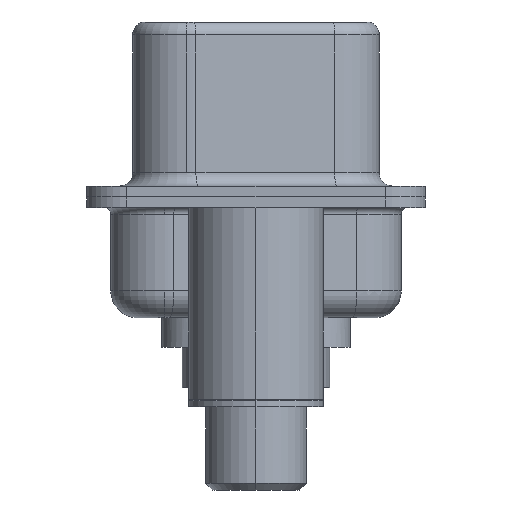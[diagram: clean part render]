
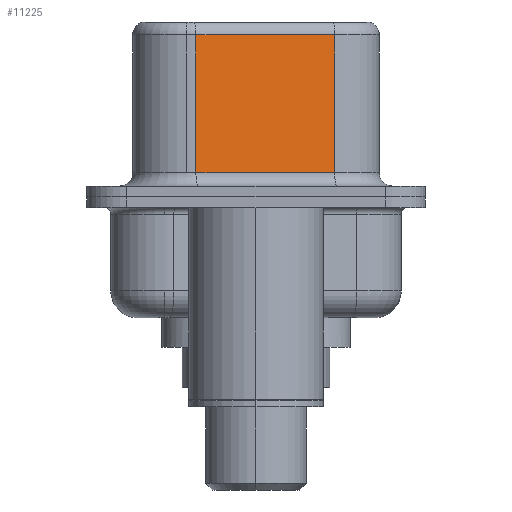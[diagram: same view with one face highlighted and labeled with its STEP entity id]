
A CAD part, left-side view. The second image highlights one B-rep face of the part: STEP entity #11225.
In plain terms, the highlighted planar face has unit normal (-0.985, -0.174, 0).
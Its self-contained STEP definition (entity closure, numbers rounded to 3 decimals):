
#11 = ORIENTED_EDGE ( 'NONE', *, *, #8225, .T. ) ;
#1440 = CARTESIAN_POINT ( 'NONE',  ( 4.565, -2.927, 0.9 ) ) ;
#1523 = VERTEX_POINT ( 'NONE', #1440 ) ;
#1738 = LINE ( 'NONE', #8258, #13459 ) ;
#1987 = LINE ( 'NONE', #2296, #6520 ) ;
#2296 = CARTESIAN_POINT ( 'NONE',  ( 4.565, -2.927, 0.9 ) ) ;
#2540 = DIRECTION ( 'NONE',  ( 0.174, -0.985, 0. ) ) ;
#2608 = ORIENTED_EDGE ( 'NONE', *, *, #13406, .F. ) ;
#2760 = DIRECTION ( 'NONE',  ( 0.985, 0.174, 0. ) ) ;
#3518 = ORIENTED_EDGE ( 'NONE', *, *, #7073, .T. ) ;
#3763 = LINE ( 'NONE', #16805, #7752 ) ;
#4968 = DIRECTION ( 'NONE',  ( -0.174, 0.985, 0. ) ) ;
#6520 = VECTOR ( 'NONE', #2540, 1000. ) ;
#7073 = EDGE_CURVE ( 'NONE', #12951, #16040, #1738, .T. ) ;
#7523 = CARTESIAN_POINT ( 'NONE',  ( 4.565, -2.927, 6.02 ) ) ;
#7752 = VECTOR ( 'NONE', #13826, 1000. ) ;
#8225 = EDGE_CURVE ( 'NONE', #17977, #1523, #1987, .T. ) ;
#8258 = CARTESIAN_POINT ( 'NONE',  ( 4.565, -2.927, 6.02 ) ) ;
#8454 = DIRECTION ( 'NONE',  ( 0., 0., -1. ) ) ;
#9390 = VECTOR ( 'NONE', #8454, 1000. ) ;
#10786 = CARTESIAN_POINT ( 'NONE',  ( 3.655, 2.233, 6.02 ) ) ;
#10844 = CARTESIAN_POINT ( 'NONE',  ( 3.655, 2.233, 0.9 ) ) ;
#11225 = ADVANCED_FACE ( 'NONE', ( #11683 ), #19380, .F. ) ;
#11683 = FACE_OUTER_BOUND ( 'NONE', #16296, .T. ) ;
#12951 = VERTEX_POINT ( 'NONE', #7523 ) ;
#12987 = LINE ( 'NONE', #19144, #9390 ) ;
#13177 = AXIS2_PLACEMENT_3D ( 'NONE', #16408, #2760, #13427 ) ;
#13406 = EDGE_CURVE ( 'NONE', #12951, #1523, #3763, .T. ) ;
#13427 = DIRECTION ( 'NONE',  ( -0.174, 0.985, 0. ) ) ;
#13459 = VECTOR ( 'NONE', #4968, 1000. ) ;
#13826 = DIRECTION ( 'NONE',  ( 0., 0., -1. ) ) ;
#14541 = ORIENTED_EDGE ( 'NONE', *, *, #16393, .T. ) ;
#16040 = VERTEX_POINT ( 'NONE', #10786 ) ;
#16296 = EDGE_LOOP ( 'NONE', ( #2608, #3518, #14541, #11 ) ) ;
#16393 = EDGE_CURVE ( 'NONE', #16040, #17977, #12987, .T. ) ;
#16408 = CARTESIAN_POINT ( 'NONE',  ( 4.565, -2.927, 6.52 ) ) ;
#16805 = CARTESIAN_POINT ( 'NONE',  ( 4.565, -2.927, 6.52 ) ) ;
#17977 = VERTEX_POINT ( 'NONE', #10844 ) ;
#19144 = CARTESIAN_POINT ( 'NONE',  ( 3.655, 2.233, 6.52 ) ) ;
#19380 = PLANE ( 'NONE',  #13177 ) ;
